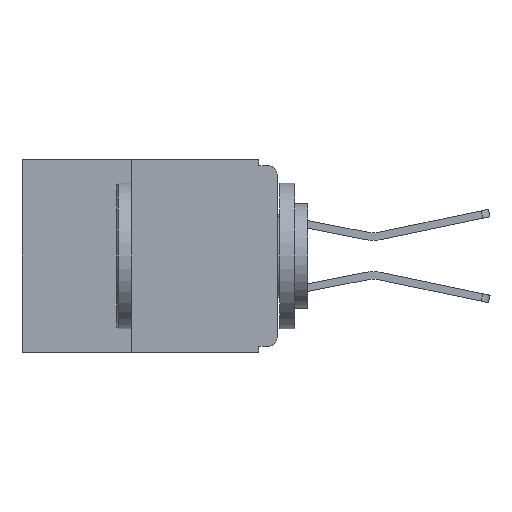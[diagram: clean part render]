
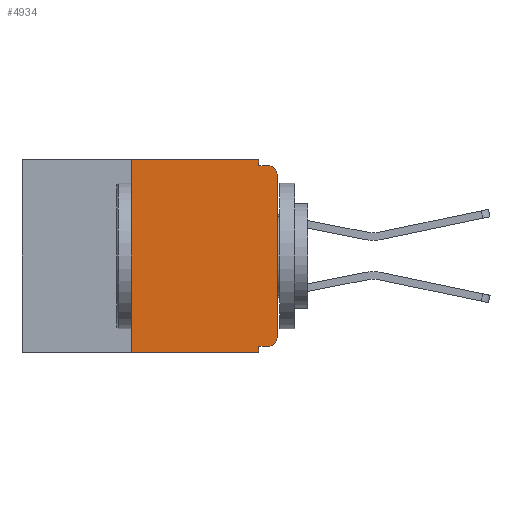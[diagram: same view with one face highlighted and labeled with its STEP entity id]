
A CAD part, left-side view. The second image highlights one B-rep face of the part: STEP entity #4934.
In plain terms, the highlighted planar face has unit normal (-1, 0, 0).
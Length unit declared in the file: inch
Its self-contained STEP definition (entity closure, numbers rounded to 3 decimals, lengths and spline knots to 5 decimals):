
#105 = CARTESIAN_POINT ( 'NONE',  ( 0., 0., 0. ) ) ;
#172 = CARTESIAN_POINT ( 'NONE',  ( 0., 0.015, -0.32 ) ) ;
#214 = ORIENTED_EDGE ( 'NONE', *, *, #6596, .T. ) ;
#531 = VERTEX_POINT ( 'NONE', #172 ) ;
#697 = CARTESIAN_POINT ( 'NONE',  ( 0., 0.031, -0.33 ) ) ;
#714 = CARTESIAN_POINT ( 'NONE',  ( 0., 0.437, 0. ) ) ;
#753 = VERTEX_POINT ( 'NONE', #6207 ) ;
#862 = VECTOR ( 'NONE', #8271, 39.37008 ) ;
#879 = PLANE ( 'NONE',  #11583 ) ;
#964 = VERTEX_POINT ( 'NONE', #11160 ) ;
#1149 = VERTEX_POINT ( 'NONE', #7797 ) ;
#1287 = CARTESIAN_POINT ( 'NONE',  ( 0., 0.031, -0.33 ) ) ;
#1330 = DIRECTION ( 'NONE',  ( 0., 0., -1. ) ) ;
#1338 = CARTESIAN_POINT ( 'NONE',  ( 0., 0., -0.32 ) ) ;
#1482 = LINE ( 'NONE', #11970, #10902 ) ;
#1560 = VERTEX_POINT ( 'NONE', #6202 ) ;
#1586 = CARTESIAN_POINT ( 'NONE',  ( 0., 0.437, -0.33 ) ) ;
#1993 = DIRECTION ( 'NONE',  ( 0., 0., -1. ) ) ;
#2154 = DIRECTION ( 'NONE',  ( 0., -1., 0. ) ) ;
#2285 = EDGE_CURVE ( 'NONE', #531, #5472, #7290, .T. ) ;
#2583 = VECTOR ( 'NONE', #2154, 39.37008 ) ;
#2741 = ORIENTED_EDGE ( 'NONE', *, *, #5216, .T. ) ;
#3259 = VERTEX_POINT ( 'NONE', #3438 ) ;
#3290 = EDGE_CURVE ( 'NONE', #3259, #4275, #10135, .T. ) ;
#3318 = ORIENTED_EDGE ( 'NONE', *, *, #2285, .F. ) ;
#3438 = CARTESIAN_POINT ( 'NONE',  ( 0., 0., -0.025 ) ) ;
#3675 = DIRECTION ( 'NONE',  ( 0., -1., 0. ) ) ;
#3807 = LINE ( 'NONE', #105, #5470 ) ;
#3875 = EDGE_CURVE ( 'NONE', #1560, #3259, #3807, .T. ) ;
#4275 = VERTEX_POINT ( 'NONE', #10744 ) ;
#4678 = DIRECTION ( 'NONE',  ( 0., 1., 0. ) ) ;
#4775 = ORIENTED_EDGE ( 'NONE', *, *, #6391, .F. ) ;
#4934 = ADVANCED_FACE ( 'NONE', ( #8423 ), #879, .F. ) ;
#5201 = ORIENTED_EDGE ( 'NONE', *, *, #7901, .F. ) ;
#5216 = EDGE_CURVE ( 'NONE', #531, #1560, #8563, .T. ) ;
#5276 = LINE ( 'NONE', #1287, #8416 ) ;
#5470 = VECTOR ( 'NONE', #5503, 39.37008 ) ;
#5472 = VERTEX_POINT ( 'NONE', #6180 ) ;
#5503 = DIRECTION ( 'NONE',  ( 0., 0., 1. ) ) ;
#6180 = CARTESIAN_POINT ( 'NONE',  ( 0., 0.031, -0.32 ) ) ;
#6202 = CARTESIAN_POINT ( 'NONE',  ( 0., 0., -0.305 ) ) ;
#6207 = CARTESIAN_POINT ( 'NONE',  ( 0., 0.031, -0.01 ) ) ;
#6329 = DIRECTION ( 'NONE',  ( -1., 0., 0. ) ) ;
#6391 = EDGE_CURVE ( 'NONE', #5472, #11142, #5276, .T. ) ;
#6395 = LINE ( 'NONE', #714, #11260 ) ;
#6409 = VECTOR ( 'NONE', #4678, 39.37008 ) ;
#6596 = EDGE_CURVE ( 'NONE', #10568, #11142, #7969, .T. ) ;
#7290 = LINE ( 'NONE', #1338, #6409 ) ;
#7487 = DIRECTION ( 'NONE',  ( 0., 0., -1. ) ) ;
#7502 = EDGE_CURVE ( 'NONE', #753, #4275, #7661, .T. ) ;
#7661 = LINE ( 'NONE', #7850, #2583 ) ;
#7769 = DIRECTION ( 'NONE',  ( 0., 0., -1. ) ) ;
#7774 = DIRECTION ( 'NONE',  ( -1., 0., 0. ) ) ;
#7781 = CARTESIAN_POINT ( 'NONE',  ( 0., 0.015, -0.305 ) ) ;
#7797 = CARTESIAN_POINT ( 'NONE',  ( 0., 0.031, 0. ) ) ;
#7850 = CARTESIAN_POINT ( 'NONE',  ( 0., 0., -0.01 ) ) ;
#7901 = EDGE_CURVE ( 'NONE', #10568, #964, #1482, .T. ) ;
#7969 = LINE ( 'NONE', #1586, #862 ) ;
#8271 = DIRECTION ( 'NONE',  ( 0., -1., 0. ) ) ;
#8416 = VECTOR ( 'NONE', #1330, 39.37008 ) ;
#8423 = FACE_OUTER_BOUND ( 'NONE', #11983, .T. ) ;
#8563 = CIRCLE ( 'NONE', #10177, 0.015 ) ;
#8643 = CARTESIAN_POINT ( 'NONE',  ( 0., 0.031, 0. ) ) ;
#8693 = EDGE_CURVE ( 'NONE', #1149, #753, #9341, .T. ) ;
#9070 = VECTOR ( 'NONE', #1993, 39.37008 ) ;
#9341 = LINE ( 'NONE', #8643, #9070 ) ;
#9353 = DIRECTION ( 'NONE',  ( 0., 0., 1. ) ) ;
#9586 = ORIENTED_EDGE ( 'NONE', *, *, #3290, .T. ) ;
#9687 = DIRECTION ( 'NONE',  ( 1., 0., 0. ) ) ;
#9794 = CARTESIAN_POINT ( 'NONE',  ( 0., 0.437, 0. ) ) ;
#10085 = CARTESIAN_POINT ( 'NONE',  ( 0., 0.015, -0.025 ) ) ;
#10135 = CIRCLE ( 'NONE', #10546, 0.015 ) ;
#10177 = AXIS2_PLACEMENT_3D ( 'NONE', #7781, #7774, #7769 ) ;
#10495 = EDGE_CURVE ( 'NONE', #964, #1149, #6395, .T. ) ;
#10546 = AXIS2_PLACEMENT_3D ( 'NONE', #10085, #6329, #7487 ) ;
#10568 = VERTEX_POINT ( 'NONE', #12084 ) ;
#10744 = CARTESIAN_POINT ( 'NONE',  ( 0., 0.015, -0.01 ) ) ;
#10798 = DIRECTION ( 'NONE',  ( 0., 0., -1. ) ) ;
#10902 = VECTOR ( 'NONE', #9353, 39.37008 ) ;
#11142 = VERTEX_POINT ( 'NONE', #697 ) ;
#11160 = CARTESIAN_POINT ( 'NONE',  ( 0., 0.25, 0. ) ) ;
#11256 = ORIENTED_EDGE ( 'NONE', *, *, #3875, .T. ) ;
#11260 = VECTOR ( 'NONE', #3675, 39.37008 ) ;
#11583 = AXIS2_PLACEMENT_3D ( 'NONE', #9794, #9687, #10798 ) ;
#11700 = ORIENTED_EDGE ( 'NONE', *, *, #8693, .F. ) ;
#11944 = ORIENTED_EDGE ( 'NONE', *, *, #7502, .F. ) ;
#11970 = CARTESIAN_POINT ( 'NONE',  ( 0., 0.25, -0.33 ) ) ;
#11972 = ORIENTED_EDGE ( 'NONE', *, *, #10495, .F. ) ;
#11983 = EDGE_LOOP ( 'NONE', ( #11256, #9586, #11944, #11700, #11972, #5201, #214, #4775, #3318, #2741 ) ) ;
#12084 = CARTESIAN_POINT ( 'NONE',  ( 0., 0.25, -0.33 ) ) ;
